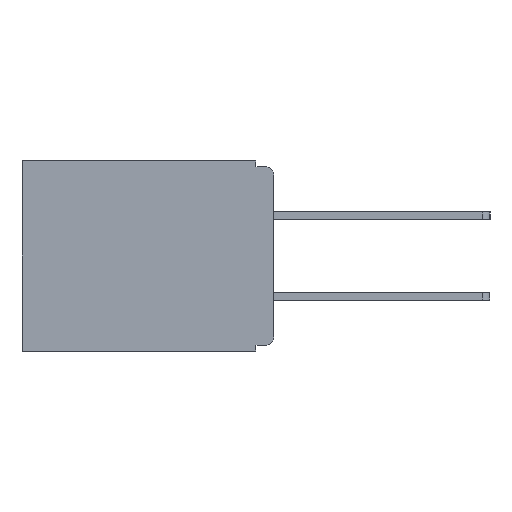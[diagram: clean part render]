
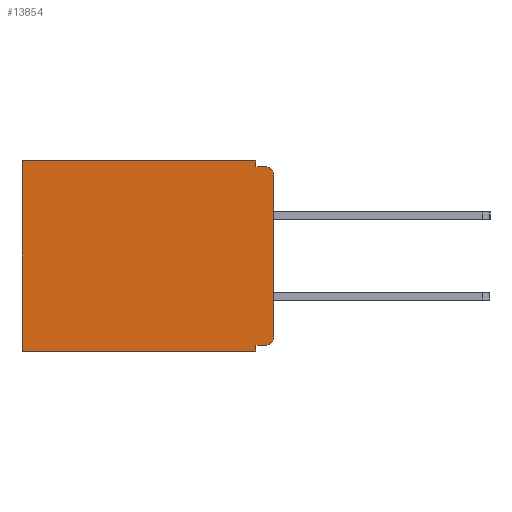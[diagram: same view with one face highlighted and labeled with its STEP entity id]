
A CAD part, left-side view. The second image highlights one B-rep face of the part: STEP entity #13854.
In plain terms, the highlighted planar face has unit normal (-1, 0, 0).
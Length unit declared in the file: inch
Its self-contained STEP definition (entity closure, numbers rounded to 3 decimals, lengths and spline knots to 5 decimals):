
#347 = ORIENTED_EDGE ( 'NONE', *, *, #22620, .T. ) ;
#362 = DIRECTION ( 'NONE',  ( 0., 0., -1. ) ) ;
#520 = CARTESIAN_POINT ( 'NONE',  ( 0.3, 0.031, -0.32 ) ) ;
#897 = VECTOR ( 'NONE', #13183, 39.37008 ) ;
#1170 = CARTESIAN_POINT ( 'NONE',  ( 0.3, 0., -0.025 ) ) ;
#2095 = EDGE_CURVE ( 'NONE', #5819, #8601, #22165, .T. ) ;
#2335 = ORIENTED_EDGE ( 'NONE', *, *, #24879, .F. ) ;
#2616 = VECTOR ( 'NONE', #4348, 39.37008 ) ;
#2984 = LINE ( 'NONE', #4548, #8023 ) ;
#3336 = CARTESIAN_POINT ( 'NONE',  ( 0.3, 0.437, 0. ) ) ;
#3431 = DIRECTION ( 'NONE',  ( -1., 0., 0. ) ) ;
#3523 = CARTESIAN_POINT ( 'NONE',  ( 0.3, 0.015, -0.025 ) ) ;
#3884 = CARTESIAN_POINT ( 'NONE',  ( 0.3, 0.031, -0.33 ) ) ;
#4348 = DIRECTION ( 'NONE',  ( 0., 0., -1. ) ) ;
#4466 = CARTESIAN_POINT ( 'NONE',  ( 0.3, 0., 0. ) ) ;
#4548 = CARTESIAN_POINT ( 'NONE',  ( 0.3, 0.031, 0. ) ) ;
#4643 = VERTEX_POINT ( 'NONE', #3884 ) ;
#4650 = VECTOR ( 'NONE', #19751, 39.37008 ) ;
#4859 = PLANE ( 'NONE',  #19626 ) ;
#5558 = DIRECTION ( 'NONE',  ( 0., 0., -1. ) ) ;
#5796 = ORIENTED_EDGE ( 'NONE', *, *, #2095, .F. ) ;
#5819 = VERTEX_POINT ( 'NONE', #11712 ) ;
#5833 = EDGE_CURVE ( 'NONE', #4643, #7786, #23391, .T. ) ;
#5965 = CARTESIAN_POINT ( 'NONE',  ( 0.3, 0.437, -0.33 ) ) ;
#6674 = VECTOR ( 'NONE', #18284, 39.37008 ) ;
#6738 = EDGE_LOOP ( 'NONE', ( #14753, #24097, #7672, #2335, #8292, #7034, #22249, #16898, #5796, #347 ) ) ;
#6826 = DIRECTION ( 'NONE',  ( 1., 0., 0. ) ) ;
#7033 = VERTEX_POINT ( 'NONE', #23326 ) ;
#7034 = ORIENTED_EDGE ( 'NONE', *, *, #14828, .T. ) ;
#7143 = CARTESIAN_POINT ( 'NONE',  ( 0.3, 0., -0.33 ) ) ;
#7397 = DIRECTION ( 'NONE',  ( 0., 1., 0. ) ) ;
#7487 = EDGE_CURVE ( 'NONE', #24979, #18466, #16807, .T. ) ;
#7596 = VECTOR ( 'NONE', #7397, 39.37008 ) ;
#7672 = ORIENTED_EDGE ( 'NONE', *, *, #7487, .F. ) ;
#7786 = VERTEX_POINT ( 'NONE', #20937 ) ;
#8023 = VECTOR ( 'NONE', #362, 39.37008 ) ;
#8292 = ORIENTED_EDGE ( 'NONE', *, *, #17159, .T. ) ;
#8326 = CARTESIAN_POINT ( 'NONE',  ( 0.3, 0.031, -0.33 ) ) ;
#8444 = VECTOR ( 'NONE', #17133, 39.37008 ) ;
#8601 = VERTEX_POINT ( 'NONE', #520 ) ;
#9038 = LINE ( 'NONE', #7143, #8444 ) ;
#9186 = LINE ( 'NONE', #8326, #2616 ) ;
#10947 = VECTOR ( 'NONE', #24929, 39.37008 ) ;
#11089 = CIRCLE ( 'NONE', #13605, 0.015 ) ;
#11684 = CARTESIAN_POINT ( 'NONE',  ( 0.3, 0., -0.33 ) ) ;
#11712 = CARTESIAN_POINT ( 'NONE',  ( 0.3, 0.015, -0.32 ) ) ;
#12779 = EDGE_CURVE ( 'NONE', #21938, #7033, #9038, .T. ) ;
#13183 = DIRECTION ( 'NONE',  ( 0., 1., 0. ) ) ;
#13380 = VERTEX_POINT ( 'NONE', #24922 ) ;
#13605 = AXIS2_PLACEMENT_3D ( 'NONE', #3523, #17358, #5558 ) ;
#13774 = CARTESIAN_POINT ( 'NONE',  ( 0.3, 0., -0.01 ) ) ;
#13854 = ADVANCED_FACE ( 'NONE', ( #17943 ), #4859, .F. ) ;
#14621 = VERTEX_POINT ( 'NONE', #3336 ) ;
#14753 = ORIENTED_EDGE ( 'NONE', *, *, #12779, .F. ) ;
#14828 = EDGE_CURVE ( 'NONE', #14621, #7786, #21694, .T. ) ;
#15258 = CARTESIAN_POINT ( 'NONE',  ( 0.3, 0.015, -0.305 ) ) ;
#16693 = CARTESIAN_POINT ( 'NONE',  ( 0.3, 0.031, -0.01 ) ) ;
#16807 = LINE ( 'NONE', #13774, #10947 ) ;
#16898 = ORIENTED_EDGE ( 'NONE', *, *, #23569, .F. ) ;
#17133 = DIRECTION ( 'NONE',  ( 0., 0., -1. ) ) ;
#17159 = EDGE_CURVE ( 'NONE', #13380, #14621, #21874, .T. ) ;
#17267 = DIRECTION ( 'NONE',  ( 0., 0., -1. ) ) ;
#17358 = DIRECTION ( 'NONE',  ( -1., 0., 0. ) ) ;
#17943 = FACE_OUTER_BOUND ( 'NONE', #6738, .T. ) ;
#18058 = AXIS2_PLACEMENT_3D ( 'NONE', #15258, #3431, #17267 ) ;
#18284 = DIRECTION ( 'NONE',  ( 0., 1., 0. ) ) ;
#18466 = VERTEX_POINT ( 'NONE', #24457 ) ;
#18676 = CARTESIAN_POINT ( 'NONE',  ( 0.3, 0., -0.33 ) ) ;
#19626 = AXIS2_PLACEMENT_3D ( 'NONE', #18676, #6826, #20710 ) ;
#19751 = DIRECTION ( 'NONE',  ( 0., 0., -1. ) ) ;
#20031 = CARTESIAN_POINT ( 'NONE',  ( 0.3, 0., -0.32 ) ) ;
#20710 = DIRECTION ( 'NONE',  ( 0., 0., -1. ) ) ;
#20937 = CARTESIAN_POINT ( 'NONE',  ( 0.3, 0.437, -0.33 ) ) ;
#21036 = CIRCLE ( 'NONE', #18058, 0.015 ) ;
#21694 = LINE ( 'NONE', #5965, #4650 ) ;
#21874 = LINE ( 'NONE', #4466, #6674 ) ;
#21938 = VERTEX_POINT ( 'NONE', #1170 ) ;
#22165 = LINE ( 'NONE', #20031, #897 ) ;
#22249 = ORIENTED_EDGE ( 'NONE', *, *, #5833, .F. ) ;
#22620 = EDGE_CURVE ( 'NONE', #5819, #7033, #21036, .T. ) ;
#23326 = CARTESIAN_POINT ( 'NONE',  ( 0.3, 0., -0.305 ) ) ;
#23391 = LINE ( 'NONE', #11684, #7596 ) ;
#23569 = EDGE_CURVE ( 'NONE', #8601, #4643, #9186, .T. ) ;
#24097 = ORIENTED_EDGE ( 'NONE', *, *, #25195, .T. ) ;
#24457 = CARTESIAN_POINT ( 'NONE',  ( 0.3, 0.015, -0.01 ) ) ;
#24879 = EDGE_CURVE ( 'NONE', #13380, #24979, #2984, .T. ) ;
#24922 = CARTESIAN_POINT ( 'NONE',  ( 0.3, 0.031, 0. ) ) ;
#24929 = DIRECTION ( 'NONE',  ( 0., -1., 0. ) ) ;
#24979 = VERTEX_POINT ( 'NONE', #16693 ) ;
#25195 = EDGE_CURVE ( 'NONE', #21938, #18466, #11089, .T. ) ;
